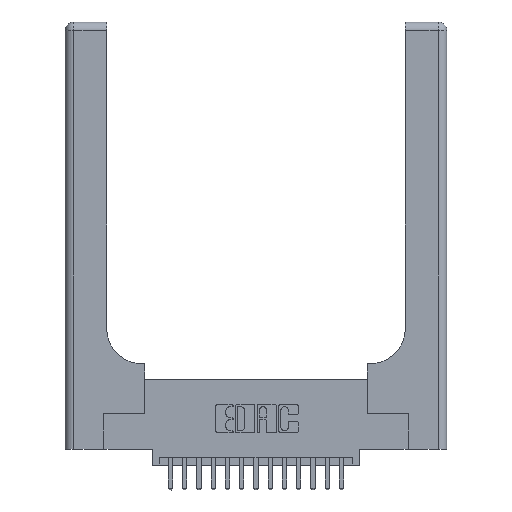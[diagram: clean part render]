
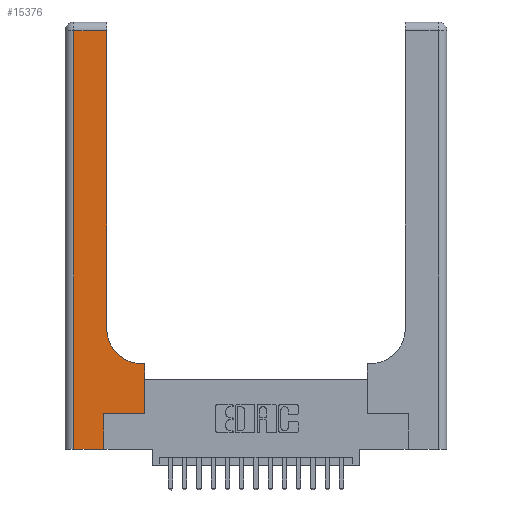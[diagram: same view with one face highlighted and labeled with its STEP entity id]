
A CAD part, top view. The second image highlights one B-rep face of the part: STEP entity #15376.
In plain terms, the highlighted planar face has unit normal (0, 0, 1).
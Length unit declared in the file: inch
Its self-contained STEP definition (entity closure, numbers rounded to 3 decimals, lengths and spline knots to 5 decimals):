
#457 = LINE ( 'NONE', #16128, #16065 ) ;
#587 = VECTOR ( 'NONE', #7278, 39.37008 ) ;
#1022 = ORIENTED_EDGE ( 'NONE', *, *, #13635, .T. ) ;
#1960 = EDGE_CURVE ( 'NONE', #14868, #13933, #12565, .T. ) ;
#2055 = ORIENTED_EDGE ( 'NONE', *, *, #17620, .T. ) ;
#2102 = CARTESIAN_POINT ( 'NONE',  ( 0.269, 0., 0.37 ) ) ;
#2355 = DIRECTION ( 'NONE',  ( -1., 0., 0. ) ) ;
#2788 = VECTOR ( 'NONE', #5777, 39.37008 ) ;
#3341 = CARTESIAN_POINT ( 'NONE',  ( 0.06, 2.94, 0.37 ) ) ;
#3371 = DIRECTION ( 'NONE',  ( -1., 0., 0. ) ) ;
#3751 = CARTESIAN_POINT ( 'NONE',  ( 0.06, 0., 0.37 ) ) ;
#4038 = EDGE_CURVE ( 'NONE', #16238, #9575, #16972, .T. ) ;
#4113 = CARTESIAN_POINT ( 'NONE',  ( 0.2915, 3., 0.37 ) ) ;
#5331 = CARTESIAN_POINT ( 'NONE',  ( 0.2915, 0.85, 0.37 ) ) ;
#5777 = DIRECTION ( 'NONE',  ( 0., 1., 0. ) ) ;
#5811 = VERTEX_POINT ( 'NONE', #5331 ) ;
#6033 = VERTEX_POINT ( 'NONE', #7353 ) ;
#6054 = EDGE_LOOP ( 'NONE', ( #1022, #13081, #10136, #17565, #16468, #16986, #11700, #2055, #7951 ) ) ;
#6401 = DIRECTION ( 'NONE',  ( -1., 0., 0. ) ) ;
#6710 = DIRECTION ( 'NONE',  ( 1., 0., 0. ) ) ;
#7278 = DIRECTION ( 'NONE',  ( 0., 1., 0. ) ) ;
#7353 = CARTESIAN_POINT ( 'NONE',  ( 0.2915, 2.94, 0.37 ) ) ;
#7691 = CARTESIAN_POINT ( 'NONE',  ( 0.06, 3., 0.37 ) ) ;
#7951 = ORIENTED_EDGE ( 'NONE', *, *, #18345, .T. ) ;
#7977 = EDGE_CURVE ( 'NONE', #13933, #11969, #14451, .T. ) ;
#9575 = VERTEX_POINT ( 'NONE', #16469 ) ;
#9618 = DIRECTION ( 'NONE',  ( 0., 1., 0. ) ) ;
#10136 = ORIENTED_EDGE ( 'NONE', *, *, #18244, .T. ) ;
#10645 = VERTEX_POINT ( 'NONE', #16249 ) ;
#11003 = EDGE_CURVE ( 'NONE', #6033, #18143, #15808, .T. ) ;
#11037 = PLANE ( 'NONE',  #11953 ) ;
#11400 = CARTESIAN_POINT ( 'NONE',  ( 0., 2.94, 0.37 ) ) ;
#11700 = ORIENTED_EDGE ( 'NONE', *, *, #4038, .T. ) ;
#11926 = CIRCLE ( 'NONE', #18664, 0.25 ) ;
#11953 = AXIS2_PLACEMENT_3D ( 'NONE', #13871, #15422, #3371 ) ;
#11969 = VERTEX_POINT ( 'NONE', #18469 ) ;
#12488 = CARTESIAN_POINT ( 'NONE',  ( 0., 0., 0.37 ) ) ;
#12565 = LINE ( 'NONE', #12488, #13279 ) ;
#13081 = ORIENTED_EDGE ( 'NONE', *, *, #11003, .T. ) ;
#13279 = VECTOR ( 'NONE', #15505, 39.37008 ) ;
#13635 = EDGE_CURVE ( 'NONE', #5811, #6033, #18762, .T. ) ;
#13871 = CARTESIAN_POINT ( 'NONE',  ( 0., 3., 0.37 ) ) ;
#13933 = VERTEX_POINT ( 'NONE', #18449 ) ;
#14105 = DIRECTION ( 'NONE',  ( 0., 0., -1. ) ) ;
#14167 = CARTESIAN_POINT ( 'NONE',  ( 0.5415, 0.85, 0.37 ) ) ;
#14451 = LINE ( 'NONE', #2102, #16117 ) ;
#14715 = CARTESIAN_POINT ( 'NONE',  ( 0.5585, 0.25, 0.37 ) ) ;
#14868 = VERTEX_POINT ( 'NONE', #3751 ) ;
#15030 = CARTESIAN_POINT ( 'NONE',  ( 0.5585, 0.25, 0.37 ) ) ;
#15082 = VECTOR ( 'NONE', #2355, 39.37008 ) ;
#15376 = ADVANCED_FACE ( 'NONE', ( #15431 ), #11037, .F. ) ;
#15422 = DIRECTION ( 'NONE',  ( 0., 0., -1. ) ) ;
#15431 = FACE_OUTER_BOUND ( 'NONE', #6054, .T. ) ;
#15505 = DIRECTION ( 'NONE',  ( 1., 0., 0. ) ) ;
#15808 = LINE ( 'NONE', #11400, #15082 ) ;
#15948 = DIRECTION ( 'NONE',  ( 1., 0., 0. ) ) ;
#16065 = VECTOR ( 'NONE', #15948, 39.37008 ) ;
#16117 = VECTOR ( 'NONE', #9618, 39.37008 ) ;
#16128 = CARTESIAN_POINT ( 'NONE',  ( 0.269, 0.25, 0.37 ) ) ;
#16238 = VERTEX_POINT ( 'NONE', #15030 ) ;
#16249 = CARTESIAN_POINT ( 'NONE',  ( 0.5415, 0.6, 0.37 ) ) ;
#16468 = ORIENTED_EDGE ( 'NONE', *, *, #7977, .T. ) ;
#16469 = CARTESIAN_POINT ( 'NONE',  ( 0.5585, 0.6, 0.37 ) ) ;
#16948 = DIRECTION ( 'NONE',  ( 0., -1., 0. ) ) ;
#16964 = CARTESIAN_POINT ( 'NONE',  ( 0.2915, 0.6, 0.37 ) ) ;
#16972 = LINE ( 'NONE', #14715, #2788 ) ;
#16986 = ORIENTED_EDGE ( 'NONE', *, *, #17258, .T. ) ;
#17258 = EDGE_CURVE ( 'NONE', #11969, #16238, #457, .T. ) ;
#17435 = LINE ( 'NONE', #16964, #18157 ) ;
#17565 = ORIENTED_EDGE ( 'NONE', *, *, #1960, .T. ) ;
#17620 = EDGE_CURVE ( 'NONE', #9575, #10645, #17435, .T. ) ;
#18097 = LINE ( 'NONE', #7691, #19492 ) ;
#18143 = VERTEX_POINT ( 'NONE', #3341 ) ;
#18157 = VECTOR ( 'NONE', #6401, 39.37008 ) ;
#18244 = EDGE_CURVE ( 'NONE', #18143, #14868, #18097, .T. ) ;
#18345 = EDGE_CURVE ( 'NONE', #10645, #5811, #11926, .T. ) ;
#18449 = CARTESIAN_POINT ( 'NONE',  ( 0.269, 0., 0.37 ) ) ;
#18469 = CARTESIAN_POINT ( 'NONE',  ( 0.269, 0.25, 0.37 ) ) ;
#18664 = AXIS2_PLACEMENT_3D ( 'NONE', #14167, #14105, #6710 ) ;
#18762 = LINE ( 'NONE', #4113, #587 ) ;
#19492 = VECTOR ( 'NONE', #16948, 39.37008 ) ;
